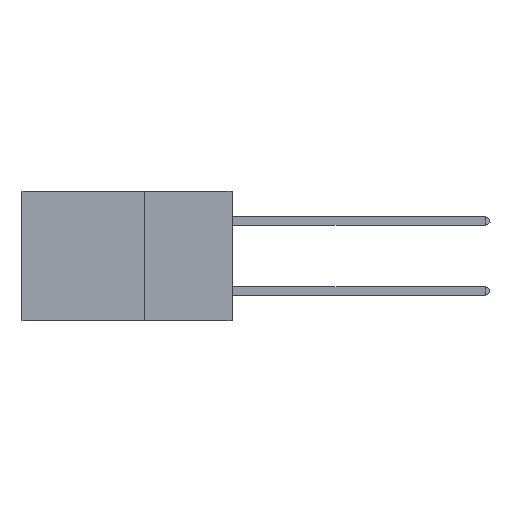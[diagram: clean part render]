
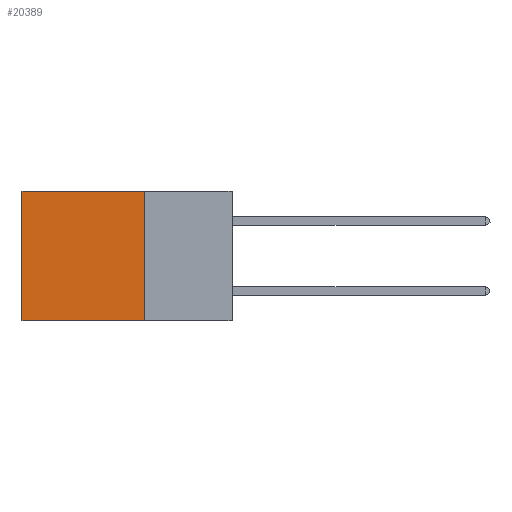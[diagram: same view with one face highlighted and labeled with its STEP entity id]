
A CAD part, left-side view. The second image highlights one B-rep face of the part: STEP entity #20389.
In plain terms, the highlighted planar face has unit normal (-1, 0, 0).
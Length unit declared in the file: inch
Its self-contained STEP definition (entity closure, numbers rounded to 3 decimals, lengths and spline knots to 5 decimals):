
#145 = EDGE_CURVE ( 'NONE', #18299, #7523, #10291, .T. ) ;
#687 = CARTESIAN_POINT ( 'NONE',  ( 0.2875, 0.25, 0. ) ) ;
#1594 = VECTOR ( 'NONE', #12529, 39.37008 ) ;
#1943 = CARTESIAN_POINT ( 'NONE',  ( 0.2875, 0.6, -0.37 ) ) ;
#2233 = ORIENTED_EDGE ( 'NONE', *, *, #6445, .T. ) ;
#3045 = CARTESIAN_POINT ( 'NONE',  ( 0.2875, 0.25, 0. ) ) ;
#3273 = CARTESIAN_POINT ( 'NONE',  ( 0.2875, 0.6, 0. ) ) ;
#4293 = VERTEX_POINT ( 'NONE', #687 ) ;
#4316 = EDGE_LOOP ( 'NONE', ( #15268, #16030, #17456, #2233 ) ) ;
#5519 = VERTEX_POINT ( 'NONE', #16829 ) ;
#6445 = EDGE_CURVE ( 'NONE', #4293, #5519, #19369, .T. ) ;
#6561 = PLANE ( 'NONE',  #18722 ) ;
#7176 = CARTESIAN_POINT ( 'NONE',  ( 0.2875, 0.25, -0.37 ) ) ;
#7523 = VERTEX_POINT ( 'NONE', #1943 ) ;
#7631 = FACE_OUTER_BOUND ( 'NONE', #4316, .T. ) ;
#7903 = VECTOR ( 'NONE', #12279, 39.37008 ) ;
#8472 = LINE ( 'NONE', #3273, #7903 ) ;
#9421 = EDGE_CURVE ( 'NONE', #4293, #18299, #22348, .T. ) ;
#10291 = LINE ( 'NONE', #7176, #22500 ) ;
#12279 = DIRECTION ( 'NONE',  ( 0., 0., -1. ) ) ;
#12529 = DIRECTION ( 'NONE',  ( 0., 0., -1. ) ) ;
#13121 = VECTOR ( 'NONE', #19306, 39.37008 ) ;
#15268 = ORIENTED_EDGE ( 'NONE', *, *, #20432, .T. ) ;
#15724 = DIRECTION ( 'NONE',  ( 0., 0., -1. ) ) ;
#16030 = ORIENTED_EDGE ( 'NONE', *, *, #145, .F. ) ;
#16212 = CARTESIAN_POINT ( 'NONE',  ( 0.2875, 0.25, 0. ) ) ;
#16829 = CARTESIAN_POINT ( 'NONE',  ( 0.2875, 0.6, 0. ) ) ;
#17179 = CARTESIAN_POINT ( 'NONE',  ( 0.2875, 0.25, -0.37 ) ) ;
#17456 = ORIENTED_EDGE ( 'NONE', *, *, #9421, .F. ) ;
#18299 = VERTEX_POINT ( 'NONE', #17179 ) ;
#18722 = AXIS2_PLACEMENT_3D ( 'NONE', #3045, #19310, #15724 ) ;
#19306 = DIRECTION ( 'NONE',  ( 0., 1., 0. ) ) ;
#19310 = DIRECTION ( 'NONE',  ( 1., 0., 0. ) ) ;
#19369 = LINE ( 'NONE', #21300, #13121 ) ;
#19636 = DIRECTION ( 'NONE',  ( 0., 1., 0. ) ) ;
#20389 = ADVANCED_FACE ( 'NONE', ( #7631 ), #6561, .F. ) ;
#20432 = EDGE_CURVE ( 'NONE', #5519, #7523, #8472, .T. ) ;
#21300 = CARTESIAN_POINT ( 'NONE',  ( 0.2875, 0.25, 0. ) ) ;
#22348 = LINE ( 'NONE', #16212, #1594 ) ;
#22500 = VECTOR ( 'NONE', #19636, 39.37008 ) ;
